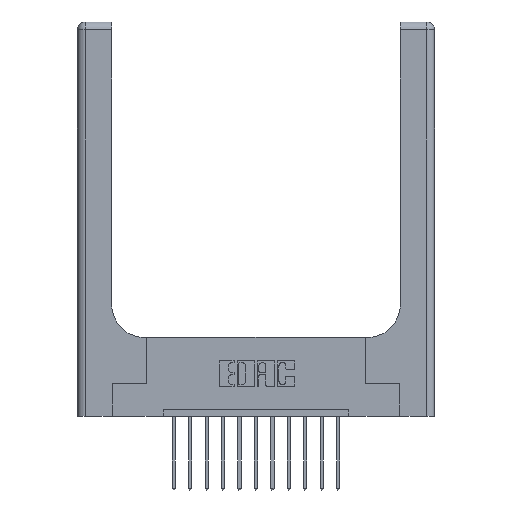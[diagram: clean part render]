
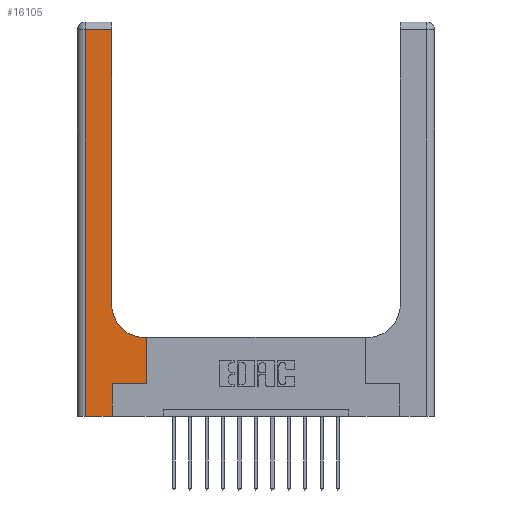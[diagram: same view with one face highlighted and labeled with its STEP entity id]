
A CAD part, top view. The second image highlights one B-rep face of the part: STEP entity #16105.
In plain terms, the highlighted planar face has unit normal (0, 0, 1).
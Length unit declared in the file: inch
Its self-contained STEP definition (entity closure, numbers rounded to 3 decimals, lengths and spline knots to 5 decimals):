
#111 = ORIENTED_EDGE ( 'NONE', *, *, #7064, .T. ) ;
#117 = DIRECTION ( 'NONE',  ( -1., 0., 0. ) ) ;
#491 = CARTESIAN_POINT ( 'NONE',  ( 0.06, 2.94, 0.37 ) ) ;
#578 = VECTOR ( 'NONE', #117, 39.37008 ) ;
#592 = DIRECTION ( 'NONE',  ( 1., 0., 0. ) ) ;
#638 = VERTEX_POINT ( 'NONE', #11938 ) ;
#677 = LINE ( 'NONE', #10902, #2956 ) ;
#848 = VERTEX_POINT ( 'NONE', #15333 ) ;
#972 = VERTEX_POINT ( 'NONE', #14589 ) ;
#1047 = VECTOR ( 'NONE', #13727, 39.37008 ) ;
#1065 = EDGE_CURVE ( 'NONE', #9979, #12623, #12318, .T. ) ;
#1168 = EDGE_CURVE ( 'NONE', #5555, #8943, #7252, .T. ) ;
#1290 = VECTOR ( 'NONE', #3577, 39.37008 ) ;
#1338 = LINE ( 'NONE', #14171, #10964 ) ;
#1366 = DIRECTION ( 'NONE',  ( 0., 0., -1. ) ) ;
#1629 = LINE ( 'NONE', #7983, #16551 ) ;
#1945 = EDGE_CURVE ( 'NONE', #14271, #15522, #1629, .T. ) ;
#2257 = CARTESIAN_POINT ( 'NONE',  ( 0.265, 0., 0.37 ) ) ;
#2906 = CARTESIAN_POINT ( 'NONE',  ( 0.26, 0.85, 0.37 ) ) ;
#2956 = VECTOR ( 'NONE', #8219, 39.37008 ) ;
#3577 = DIRECTION ( 'NONE',  ( 1., 0., 0. ) ) ;
#3693 = ORIENTED_EDGE ( 'NONE', *, *, #1065, .T. ) ;
#4912 = CARTESIAN_POINT ( 'NONE',  ( 0.528, 0.25, 0.37 ) ) ;
#5023 = DIRECTION ( 'NONE',  ( 0., 1., 0. ) ) ;
#5051 = EDGE_CURVE ( 'NONE', #638, #972, #10074, .T. ) ;
#5119 = CARTESIAN_POINT ( 'NONE',  ( 0.26, 2.94, 0.37 ) ) ;
#5128 = PLANE ( 'NONE',  #13945 ) ;
#5133 = CARTESIAN_POINT ( 'NONE',  ( 0., 0., 0.37 ) ) ;
#5370 = CARTESIAN_POINT ( 'NONE',  ( 0.528, 0.25, 0.37 ) ) ;
#5427 = ORIENTED_EDGE ( 'NONE', *, *, #8784, .T. ) ;
#5555 = VERTEX_POINT ( 'NONE', #5370 ) ;
#5712 = LINE ( 'NONE', #16275, #6724 ) ;
#5786 = ORIENTED_EDGE ( 'NONE', *, *, #15432, .T. ) ;
#6469 = CARTESIAN_POINT ( 'NONE',  ( 0.51, 0.6, 0.37 ) ) ;
#6607 = CARTESIAN_POINT ( 'NONE',  ( 0.26, 0.6, 0.37 ) ) ;
#6724 = VECTOR ( 'NONE', #592, 39.37008 ) ;
#6731 = DIRECTION ( 'NONE',  ( -1., 0., 0. ) ) ;
#6840 = CARTESIAN_POINT ( 'NONE',  ( 0.51, 0.85, 0.37 ) ) ;
#6957 = AXIS2_PLACEMENT_3D ( 'NONE', #6840, #15937, #11984 ) ;
#7064 = EDGE_CURVE ( 'NONE', #15522, #638, #677, .T. ) ;
#7252 = LINE ( 'NONE', #4912, #1047 ) ;
#7632 = ORIENTED_EDGE ( 'NONE', *, *, #10200, .T. ) ;
#7892 = VECTOR ( 'NONE', #8604, 39.37008 ) ;
#7983 = CARTESIAN_POINT ( 'NONE',  ( 0., 2.94, 0.37 ) ) ;
#8219 = DIRECTION ( 'NONE',  ( 0., -1., 0. ) ) ;
#8604 = DIRECTION ( 'NONE',  ( 0., 1., 0. ) ) ;
#8784 = EDGE_CURVE ( 'NONE', #8943, #9979, #14250, .T. ) ;
#8943 = VERTEX_POINT ( 'NONE', #9530 ) ;
#9230 = FACE_OUTER_BOUND ( 'NONE', #12128, .T. ) ;
#9530 = CARTESIAN_POINT ( 'NONE',  ( 0.528, 0.6, 0.37 ) ) ;
#9781 = ORIENTED_EDGE ( 'NONE', *, *, #14416, .T. ) ;
#9787 = ORIENTED_EDGE ( 'NONE', *, *, #5051, .T. ) ;
#9979 = VERTEX_POINT ( 'NONE', #6469 ) ;
#10074 = LINE ( 'NONE', #5133, #1290 ) ;
#10200 = EDGE_CURVE ( 'NONE', #848, #5555, #5712, .T. ) ;
#10259 = ORIENTED_EDGE ( 'NONE', *, *, #1945, .T. ) ;
#10902 = CARTESIAN_POINT ( 'NONE',  ( 0.06, 3., 0.37 ) ) ;
#10964 = VECTOR ( 'NONE', #5023, 39.37008 ) ;
#11938 = CARTESIAN_POINT ( 'NONE',  ( 0.06, 0., 0.37 ) ) ;
#11984 = DIRECTION ( 'NONE',  ( 1., 0., 0. ) ) ;
#12128 = EDGE_LOOP ( 'NONE', ( #5786, #10259, #111, #9787, #9781, #7632, #12953, #5427, #3693 ) ) ;
#12318 = CIRCLE ( 'NONE', #6957, 0.25 ) ;
#12623 = VERTEX_POINT ( 'NONE', #2906 ) ;
#12953 = ORIENTED_EDGE ( 'NONE', *, *, #1168, .T. ) ;
#13727 = DIRECTION ( 'NONE',  ( 0., 1., 0. ) ) ;
#13746 = LINE ( 'NONE', #2257, #7892 ) ;
#13945 = AXIS2_PLACEMENT_3D ( 'NONE', #15380, #1366, #6731 ) ;
#14171 = CARTESIAN_POINT ( 'NONE',  ( 0.26, 3., 0.37 ) ) ;
#14250 = LINE ( 'NONE', #6607, #578 ) ;
#14271 = VERTEX_POINT ( 'NONE', #5119 ) ;
#14416 = EDGE_CURVE ( 'NONE', #972, #848, #13746, .T. ) ;
#14589 = CARTESIAN_POINT ( 'NONE',  ( 0.265, 0., 0.37 ) ) ;
#15333 = CARTESIAN_POINT ( 'NONE',  ( 0.265, 0.25, 0.37 ) ) ;
#15380 = CARTESIAN_POINT ( 'NONE',  ( 0., 3., 0.37 ) ) ;
#15432 = EDGE_CURVE ( 'NONE', #12623, #14271, #1338, .T. ) ;
#15522 = VERTEX_POINT ( 'NONE', #491 ) ;
#15636 = DIRECTION ( 'NONE',  ( -1., 0., 0. ) ) ;
#15937 = DIRECTION ( 'NONE',  ( 0., 0., -1. ) ) ;
#16105 = ADVANCED_FACE ( 'NONE', ( #9230 ), #5128, .F. ) ;
#16275 = CARTESIAN_POINT ( 'NONE',  ( 0.265, 0.25, 0.37 ) ) ;
#16551 = VECTOR ( 'NONE', #15636, 39.37008 ) ;
